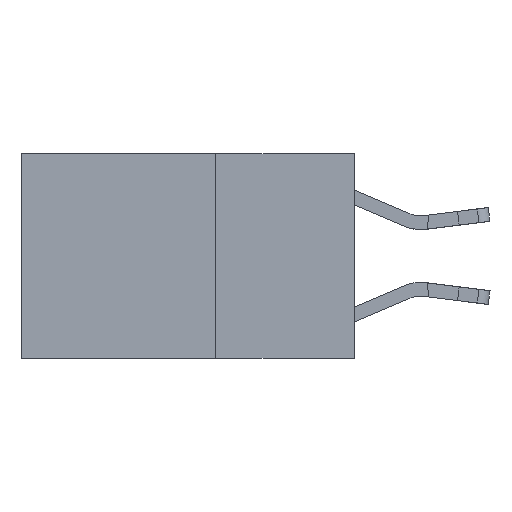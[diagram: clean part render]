
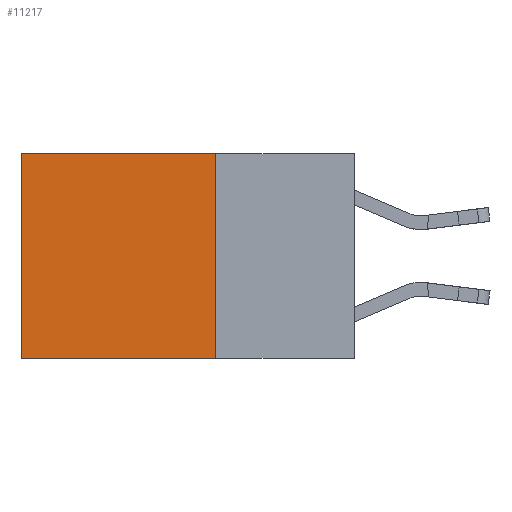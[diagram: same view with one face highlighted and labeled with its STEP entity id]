
A CAD part, left-side view. The second image highlights one B-rep face of the part: STEP entity #11217.
In plain terms, the highlighted planar face has unit normal (-1, 0, 0).
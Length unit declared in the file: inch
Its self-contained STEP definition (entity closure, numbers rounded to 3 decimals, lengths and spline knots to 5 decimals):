
#1255 = LINE ( 'NONE', #7499, #13247 ) ;
#1318 = DIRECTION ( 'NONE',  ( 0., 0., -1. ) ) ;
#2689 = EDGE_CURVE ( 'NONE', #3604, #21288, #1255, .T. ) ;
#2780 = VERTEX_POINT ( 'NONE', #12298 ) ;
#2824 = CARTESIAN_POINT ( 'NONE',  ( 0.2625, 0.6, 0. ) ) ;
#3604 = VERTEX_POINT ( 'NONE', #2824 ) ;
#4039 = EDGE_CURVE ( 'NONE', #2780, #21288, #16628, .T. ) ;
#5875 = ORIENTED_EDGE ( 'NONE', *, *, #4039, .F. ) ;
#6103 = EDGE_CURVE ( 'NONE', #20497, #3604, #14301, .T. ) ;
#7498 = LINE ( 'NONE', #12944, #8584 ) ;
#7499 = CARTESIAN_POINT ( 'NONE',  ( 0.2625, 0.6, 0. ) ) ;
#8584 = VECTOR ( 'NONE', #13013, 39.37008 ) ;
#10427 = DIRECTION ( 'NONE',  ( 0., 0., -1. ) ) ;
#10569 = CARTESIAN_POINT ( 'NONE',  ( 0.2625, 0.25, 0. ) ) ;
#11053 = VECTOR ( 'NONE', #21771, 39.37008 ) ;
#11111 = CARTESIAN_POINT ( 'NONE',  ( 0.2625, 0.6, -0.37 ) ) ;
#11217 = ADVANCED_FACE ( 'NONE', ( #14130 ), #13660, .F. ) ;
#12298 = CARTESIAN_POINT ( 'NONE',  ( 0.2625, 0.25, -0.37 ) ) ;
#12944 = CARTESIAN_POINT ( 'NONE',  ( 0.2625, 0.25, 0. ) ) ;
#13013 = DIRECTION ( 'NONE',  ( 0., 0., -1. ) ) ;
#13247 = VECTOR ( 'NONE', #1318, 39.37008 ) ;
#13535 = ORIENTED_EDGE ( 'NONE', *, *, #6103, .T. ) ;
#13577 = CARTESIAN_POINT ( 'NONE',  ( 0.2625, 0.25, 0. ) ) ;
#13660 = PLANE ( 'NONE',  #19333 ) ;
#14130 = FACE_OUTER_BOUND ( 'NONE', #19965, .T. ) ;
#14301 = LINE ( 'NONE', #21920, #11053 ) ;
#14324 = DIRECTION ( 'NONE',  ( 0., 1., 0. ) ) ;
#16628 = LINE ( 'NONE', #17892, #18772 ) ;
#17246 = EDGE_CURVE ( 'NONE', #20497, #2780, #7498, .T. ) ;
#17740 = ORIENTED_EDGE ( 'NONE', *, *, #17246, .F. ) ;
#17892 = CARTESIAN_POINT ( 'NONE',  ( 0.2625, 0.25, -0.37 ) ) ;
#18534 = ORIENTED_EDGE ( 'NONE', *, *, #2689, .T. ) ;
#18772 = VECTOR ( 'NONE', #14324, 39.37008 ) ;
#19333 = AXIS2_PLACEMENT_3D ( 'NONE', #10569, #20705, #10427 ) ;
#19965 = EDGE_LOOP ( 'NONE', ( #18534, #5875, #17740, #13535 ) ) ;
#20497 = VERTEX_POINT ( 'NONE', #13577 ) ;
#20705 = DIRECTION ( 'NONE',  ( 1., 0., 0. ) ) ;
#21288 = VERTEX_POINT ( 'NONE', #11111 ) ;
#21771 = DIRECTION ( 'NONE',  ( 0., 1., 0. ) ) ;
#21920 = CARTESIAN_POINT ( 'NONE',  ( 0.2625, 0.25, 0. ) ) ;
